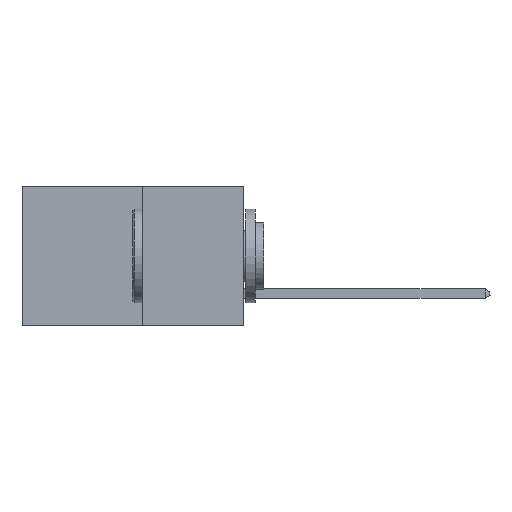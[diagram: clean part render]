
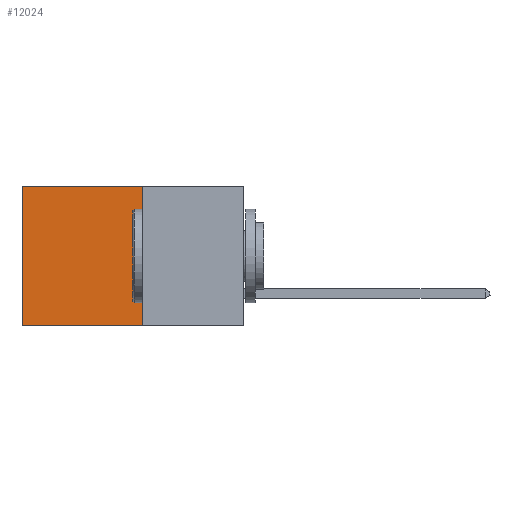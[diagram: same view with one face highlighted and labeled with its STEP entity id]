
A CAD part, left-side view. The second image highlights one B-rep face of the part: STEP entity #12024.
In plain terms, the highlighted planar face has unit normal (-1, 0, 0).
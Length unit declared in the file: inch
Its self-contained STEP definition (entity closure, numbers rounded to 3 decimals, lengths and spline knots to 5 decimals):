
#766 = EDGE_CURVE ( 'NONE', #8944, #9531, #16056, .T. ) ;
#2722 = CARTESIAN_POINT ( 'NONE',  ( 0.277, 0.59, 0. ) ) ;
#3688 = LINE ( 'NONE', #10351, #15763 ) ;
#4515 = LINE ( 'NONE', #10938, #16098 ) ;
#4998 = VECTOR ( 'NONE', #11760, 39.37008 ) ;
#5357 = DIRECTION ( 'NONE',  ( 0., 0., -1. ) ) ;
#6004 = AXIS2_PLACEMENT_3D ( 'NONE', #17168, #8216, #18670 ) ;
#6045 = EDGE_CURVE ( 'NONE', #8944, #16184, #9036, .T. ) ;
#6077 = EDGE_CURVE ( 'NONE', #16184, #13249, #4515, .T. ) ;
#6297 = CARTESIAN_POINT ( 'NONE',  ( 0.277, 0.59, -0.37 ) ) ;
#6507 = ORIENTED_EDGE ( 'NONE', *, *, #6077, .T. ) ;
#6685 = PLANE ( 'NONE',  #6004 ) ;
#7900 = ORIENTED_EDGE ( 'NONE', *, *, #9680, .F. ) ;
#8216 = DIRECTION ( 'NONE',  ( 1., 0., 0. ) ) ;
#8944 = VERTEX_POINT ( 'NONE', #17489 ) ;
#9036 = LINE ( 'NONE', #11718, #4998 ) ;
#9531 = VERTEX_POINT ( 'NONE', #18909 ) ;
#9680 = EDGE_CURVE ( 'NONE', #9531, #13249, #3688, .T. ) ;
#10351 = CARTESIAN_POINT ( 'NONE',  ( 0.277, 0.27, -0.37 ) ) ;
#10828 = DIRECTION ( 'NONE',  ( 0., 0., -1. ) ) ;
#10938 = CARTESIAN_POINT ( 'NONE',  ( 0.277, 0.59, -0.37 ) ) ;
#11718 = CARTESIAN_POINT ( 'NONE',  ( 0.277, 0.27, 0. ) ) ;
#11760 = DIRECTION ( 'NONE',  ( 0., 1., 0. ) ) ;
#11898 = DIRECTION ( 'NONE',  ( 0., 1., 0. ) ) ;
#12012 = ORIENTED_EDGE ( 'NONE', *, *, #766, .F. ) ;
#12024 = ADVANCED_FACE ( 'NONE', ( #18435 ), #6685, .F. ) ;
#12080 = VECTOR ( 'NONE', #5357, 39.37008 ) ;
#13249 = VERTEX_POINT ( 'NONE', #6297 ) ;
#15069 = CARTESIAN_POINT ( 'NONE',  ( 0.277, 0.27, -0.37 ) ) ;
#15763 = VECTOR ( 'NONE', #11898, 39.37008 ) ;
#16056 = LINE ( 'NONE', #15069, #12080 ) ;
#16098 = VECTOR ( 'NONE', #10828, 39.37008 ) ;
#16184 = VERTEX_POINT ( 'NONE', #2722 ) ;
#16484 = EDGE_LOOP ( 'NONE', ( #6507, #7900, #12012, #19224 ) ) ;
#17168 = CARTESIAN_POINT ( 'NONE',  ( 0.277, 0.27, -0.37 ) ) ;
#17489 = CARTESIAN_POINT ( 'NONE',  ( 0.277, 0.27, 0. ) ) ;
#18435 = FACE_OUTER_BOUND ( 'NONE', #16484, .T. ) ;
#18670 = DIRECTION ( 'NONE',  ( 0., 0., -1. ) ) ;
#18909 = CARTESIAN_POINT ( 'NONE',  ( 0.277, 0.27, -0.37 ) ) ;
#19224 = ORIENTED_EDGE ( 'NONE', *, *, #6045, .T. ) ;
